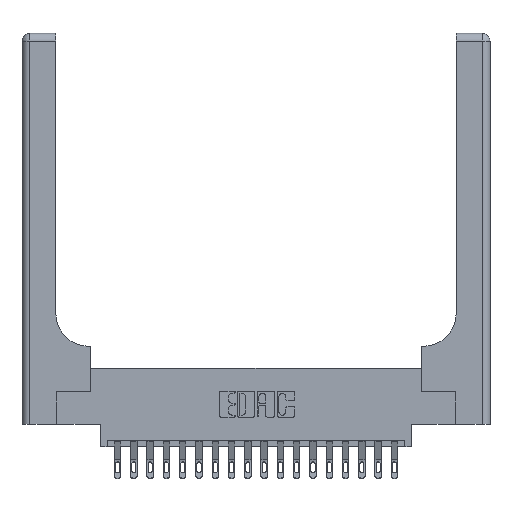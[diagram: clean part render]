
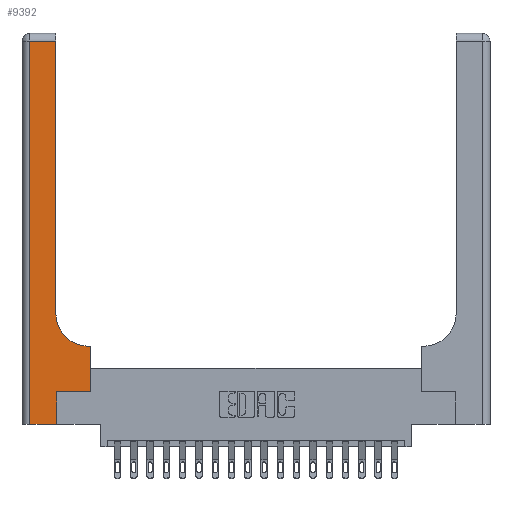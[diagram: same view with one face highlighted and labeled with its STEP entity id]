
A CAD part, top view. The second image highlights one B-rep face of the part: STEP entity #9392.
In plain terms, the highlighted planar face has unit normal (0, 0, 1).
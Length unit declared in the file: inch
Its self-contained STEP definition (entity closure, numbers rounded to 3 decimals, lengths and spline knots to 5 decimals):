
#163 = DIRECTION ( 'NONE',  ( -1., 0., 0. ) ) ;
#378 = CARTESIAN_POINT ( 'NONE',  ( 0.528, 0.25, 0.37 ) ) ;
#655 = CARTESIAN_POINT ( 'NONE',  ( 0.06, 3., 0.37 ) ) ;
#687 = LINE ( 'NONE', #655, #8803 ) ;
#755 = VECTOR ( 'NONE', #20263, 39.37008 ) ;
#933 = CARTESIAN_POINT ( 'NONE',  ( 0.265, 0., 0.37 ) ) ;
#970 = CARTESIAN_POINT ( 'NONE',  ( 0.26, 3., 0.37 ) ) ;
#1110 = EDGE_CURVE ( 'NONE', #6434, #15472, #3979, .T. ) ;
#1178 = ORIENTED_EDGE ( 'NONE', *, *, #4770, .T. ) ;
#1738 = CIRCLE ( 'NONE', #4575, 0.25 ) ;
#1860 = VECTOR ( 'NONE', #163, 39.37008 ) ;
#1958 = LINE ( 'NONE', #933, #11107 ) ;
#2414 = LINE ( 'NONE', #8012, #14728 ) ;
#2572 = DIRECTION ( 'NONE',  ( 0., 1., 0. ) ) ;
#2956 = VERTEX_POINT ( 'NONE', #18334 ) ;
#3227 = ORIENTED_EDGE ( 'NONE', *, *, #18372, .T. ) ;
#3284 = VERTEX_POINT ( 'NONE', #17591 ) ;
#3289 = VECTOR ( 'NONE', #10519, 39.37008 ) ;
#3979 = LINE ( 'NONE', #11776, #8322 ) ;
#4466 = ORIENTED_EDGE ( 'NONE', *, *, #1110, .T. ) ;
#4575 = AXIS2_PLACEMENT_3D ( 'NONE', #18111, #8648, #19683 ) ;
#4770 = EDGE_CURVE ( 'NONE', #12976, #17590, #20211, .T. ) ;
#5009 = CARTESIAN_POINT ( 'NONE',  ( 0.26, 0.6, 0.37 ) ) ;
#5595 = LINE ( 'NONE', #970, #14125 ) ;
#6324 = VERTEX_POINT ( 'NONE', #6325 ) ;
#6325 = CARTESIAN_POINT ( 'NONE',  ( 0.265, 0.25, 0.37 ) ) ;
#6434 = VERTEX_POINT ( 'NONE', #8248 ) ;
#7260 = CARTESIAN_POINT ( 'NONE',  ( 0.528, 0.25, 0.37 ) ) ;
#7399 = CARTESIAN_POINT ( 'NONE',  ( 0.26, 2.94, 0.37 ) ) ;
#7626 = EDGE_LOOP ( 'NONE', ( #15724, #20384, #12560, #4466, #17217, #9303, #1178, #14527, #3227 ) ) ;
#8012 = CARTESIAN_POINT ( 'NONE',  ( 0., 2.94, 0.37 ) ) ;
#8248 = CARTESIAN_POINT ( 'NONE',  ( 0.06, 0., 0.37 ) ) ;
#8322 = VECTOR ( 'NONE', #11732, 39.37008 ) ;
#8335 = EDGE_CURVE ( 'NONE', #17590, #2956, #19809, .T. ) ;
#8648 = DIRECTION ( 'NONE',  ( 0., 0., -1. ) ) ;
#8803 = VECTOR ( 'NONE', #19828, 39.37008 ) ;
#9303 = ORIENTED_EDGE ( 'NONE', *, *, #17493, .T. ) ;
#9392 = ADVANCED_FACE ( 'NONE', ( #9442 ), #20393, .F. ) ;
#9442 = FACE_OUTER_BOUND ( 'NONE', #7626, .T. ) ;
#9448 = DIRECTION ( 'NONE',  ( 0., 0., -1. ) ) ;
#9519 = AXIS2_PLACEMENT_3D ( 'NONE', #15737, #9448, #20458 ) ;
#9885 = LINE ( 'NONE', #12414, #755 ) ;
#10519 = DIRECTION ( 'NONE',  ( 0., 1., 0. ) ) ;
#11107 = VECTOR ( 'NONE', #2572, 39.37008 ) ;
#11170 = CARTESIAN_POINT ( 'NONE',  ( 0.528, 0.6, 0.37 ) ) ;
#11732 = DIRECTION ( 'NONE',  ( 1., 0., 0. ) ) ;
#11776 = CARTESIAN_POINT ( 'NONE',  ( 0., 0., 0.37 ) ) ;
#12314 = DIRECTION ( 'NONE',  ( 0., 1., 0. ) ) ;
#12414 = CARTESIAN_POINT ( 'NONE',  ( 0.265, 0.25, 0.37 ) ) ;
#12560 = ORIENTED_EDGE ( 'NONE', *, *, #19416, .T. ) ;
#12976 = VERTEX_POINT ( 'NONE', #378 ) ;
#13401 = EDGE_CURVE ( 'NONE', #15472, #6324, #1958, .T. ) ;
#14125 = VECTOR ( 'NONE', #12314, 39.37008 ) ;
#14527 = ORIENTED_EDGE ( 'NONE', *, *, #8335, .T. ) ;
#14728 = VECTOR ( 'NONE', #20560, 39.37008 ) ;
#15472 = VERTEX_POINT ( 'NONE', #19350 ) ;
#15724 = ORIENTED_EDGE ( 'NONE', *, *, #16947, .T. ) ;
#15737 = CARTESIAN_POINT ( 'NONE',  ( 0., 3., 0.37 ) ) ;
#16813 = CARTESIAN_POINT ( 'NONE',  ( 0.06, 2.94, 0.37 ) ) ;
#16947 = EDGE_CURVE ( 'NONE', #3284, #19521, #5595, .T. ) ;
#17217 = ORIENTED_EDGE ( 'NONE', *, *, #13401, .T. ) ;
#17493 = EDGE_CURVE ( 'NONE', #6324, #12976, #9885, .T. ) ;
#17590 = VERTEX_POINT ( 'NONE', #11170 ) ;
#17591 = CARTESIAN_POINT ( 'NONE',  ( 0.26, 0.85, 0.37 ) ) ;
#18111 = CARTESIAN_POINT ( 'NONE',  ( 0.51, 0.85, 0.37 ) ) ;
#18334 = CARTESIAN_POINT ( 'NONE',  ( 0.51, 0.6, 0.37 ) ) ;
#18372 = EDGE_CURVE ( 'NONE', #2956, #3284, #1738, .T. ) ;
#18465 = VERTEX_POINT ( 'NONE', #16813 ) ;
#19350 = CARTESIAN_POINT ( 'NONE',  ( 0.265, 0., 0.37 ) ) ;
#19416 = EDGE_CURVE ( 'NONE', #18465, #6434, #687, .T. ) ;
#19521 = VERTEX_POINT ( 'NONE', #7399 ) ;
#19683 = DIRECTION ( 'NONE',  ( 1., 0., 0. ) ) ;
#19809 = LINE ( 'NONE', #5009, #1860 ) ;
#19828 = DIRECTION ( 'NONE',  ( 0., -1., 0. ) ) ;
#20211 = LINE ( 'NONE', #7260, #3289 ) ;
#20263 = DIRECTION ( 'NONE',  ( 1., 0., 0. ) ) ;
#20384 = ORIENTED_EDGE ( 'NONE', *, *, #20473, .T. ) ;
#20393 = PLANE ( 'NONE',  #9519 ) ;
#20458 = DIRECTION ( 'NONE',  ( -1., 0., 0. ) ) ;
#20473 = EDGE_CURVE ( 'NONE', #19521, #18465, #2414, .T. ) ;
#20560 = DIRECTION ( 'NONE',  ( -1., 0., 0. ) ) ;
